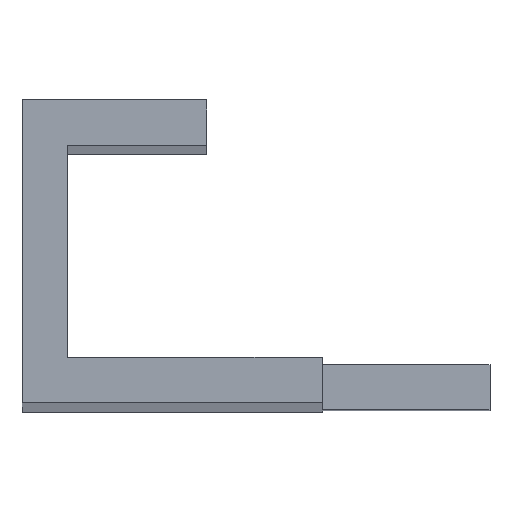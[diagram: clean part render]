
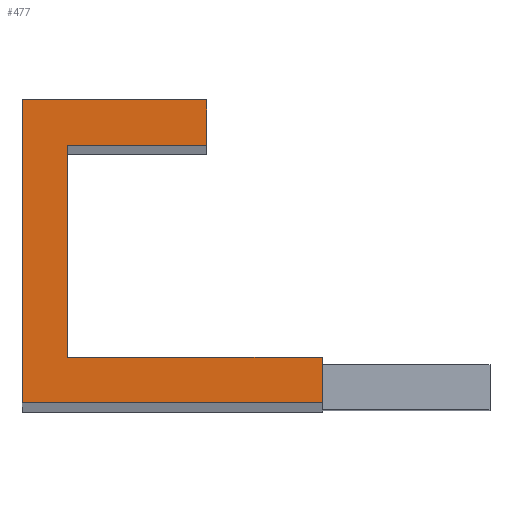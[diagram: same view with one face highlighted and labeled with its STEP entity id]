
A CAD part, top view. The second image highlights one B-rep face of the part: STEP entity #477.
In plain terms, the highlighted planar face has unit normal (0, 0, 1).
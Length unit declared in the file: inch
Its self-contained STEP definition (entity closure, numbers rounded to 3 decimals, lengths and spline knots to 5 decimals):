
#63=FACE_OUTER_BOUND('',#85,.T.);
#85=EDGE_LOOP('',(#327,#328,#329,#330,#331,#332,#333,#334));
#123=LINE('',#707,#167);
#124=LINE('',#709,#168);
#125=LINE('',#711,#169);
#126=LINE('',#713,#170);
#127=LINE('',#715,#171);
#128=LINE('',#717,#172);
#129=LINE('',#719,#173);
#130=LINE('',#720,#174);
#167=VECTOR('',#569,0.3937);
#168=VECTOR('',#570,0.3937);
#169=VECTOR('',#571,0.3937);
#170=VECTOR('',#572,0.3937);
#171=VECTOR('',#573,0.3937);
#172=VECTOR('',#574,0.3937);
#173=VECTOR('',#575,0.3937);
#174=VECTOR('',#576,0.3937);
#211=VERTEX_POINT('',#705);
#212=VERTEX_POINT('',#706);
#213=VERTEX_POINT('',#708);
#214=VERTEX_POINT('',#710);
#215=VERTEX_POINT('',#712);
#216=VERTEX_POINT('',#714);
#217=VERTEX_POINT('',#716);
#218=VERTEX_POINT('',#718);
#259=EDGE_CURVE('',#211,#212,#123,.T.);
#260=EDGE_CURVE('',#213,#211,#124,.T.);
#261=EDGE_CURVE('',#214,#213,#125,.T.);
#262=EDGE_CURVE('',#215,#214,#126,.T.);
#263=EDGE_CURVE('',#216,#215,#127,.T.);
#264=EDGE_CURVE('',#217,#216,#128,.T.);
#265=EDGE_CURVE('',#218,#217,#129,.T.);
#266=EDGE_CURVE('',#212,#218,#130,.T.);
#327=ORIENTED_EDGE('',*,*,#259,.F.);
#328=ORIENTED_EDGE('',*,*,#260,.F.);
#329=ORIENTED_EDGE('',*,*,#261,.F.);
#330=ORIENTED_EDGE('',*,*,#262,.F.);
#331=ORIENTED_EDGE('',*,*,#263,.F.);
#332=ORIENTED_EDGE('',*,*,#264,.F.);
#333=ORIENTED_EDGE('',*,*,#265,.F.);
#334=ORIENTED_EDGE('',*,*,#266,.F.);
#463=PLANE('',#519);
#477=ADVANCED_FACE('',(#63),#463,.F.);
#519=AXIS2_PLACEMENT_3D('',#704,#567,#568);
#567=DIRECTION('center_axis',(0.,0.,-1.));
#568=DIRECTION('ref_axis',(-1.,0.,0.));
#569=DIRECTION('',(0.,-1.,0.));
#570=DIRECTION('',(1.,0.,0.));
#571=DIRECTION('',(0.,-1.,0.));
#572=DIRECTION('',(-1.,0.,0.));
#573=DIRECTION('',(0.,-1.,0.));
#574=DIRECTION('',(1.,0.,0.));
#575=DIRECTION('',(0.,1.,0.));
#576=DIRECTION('',(-1.,0.,0.));
#704=CARTESIAN_POINT('Origin',(-0.195,0.19685,6.80194));
#705=CARTESIAN_POINT('',(0.,0.05906,6.80194));
#706=CARTESIAN_POINT('',(0.,0.,6.80194));
#707=CARTESIAN_POINT('',(0.,0.09843,6.80194));
#708=CARTESIAN_POINT('',(-0.33094,0.05906,6.80194));
#709=CARTESIAN_POINT('',(-0.0975,0.05906,6.80194));
#710=CARTESIAN_POINT('',(-0.33094,0.33465,6.80194));
#711=CARTESIAN_POINT('',(-0.33094,0.12795,6.80194));
#712=CARTESIAN_POINT('',(-0.15,0.33465,6.80194));
#713=CARTESIAN_POINT('',(-0.26297,0.33465,6.80194));
#714=CARTESIAN_POINT('',(-0.15,0.3937,6.80194));
#715=CARTESIAN_POINT('',(-0.15,0.29528,6.80194));
#716=CARTESIAN_POINT('',(-0.39,0.3937,6.80194));
#717=CARTESIAN_POINT('',(-0.1525,0.3937,6.80194));
#718=CARTESIAN_POINT('',(-0.39,0.,6.80194));
#719=CARTESIAN_POINT('',(-0.39,0.29528,6.80194));
#720=CARTESIAN_POINT('',(-0.2925,0.,6.80194));
